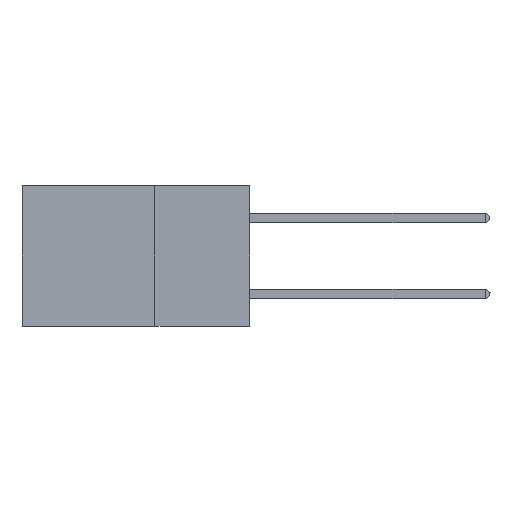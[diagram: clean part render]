
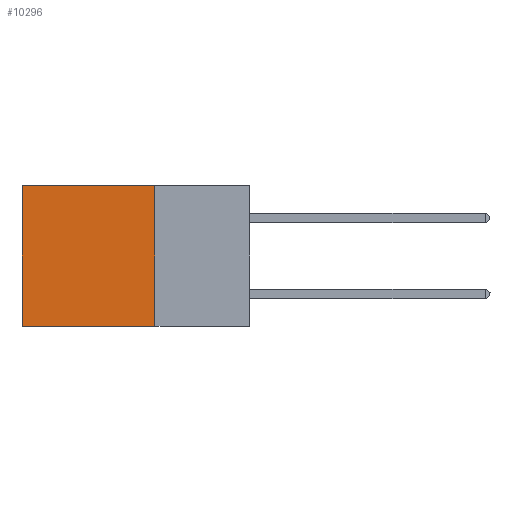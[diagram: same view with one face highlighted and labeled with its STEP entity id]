
A CAD part, left-side view. The second image highlights one B-rep face of the part: STEP entity #10296.
In plain terms, the highlighted planar face has unit normal (-1, 0, 0).
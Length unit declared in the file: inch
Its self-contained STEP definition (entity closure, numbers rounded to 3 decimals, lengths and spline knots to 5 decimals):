
#1873 = LINE ( 'NONE', #22640, #8203 ) ;
#2270 = AXIS2_PLACEMENT_3D ( 'NONE', #21658, #13284, #27161 ) ;
#2515 = CARTESIAN_POINT ( 'NONE',  ( 0.2875, 0.25, -0.37 ) ) ;
#2708 = EDGE_CURVE ( 'NONE', #6858, #5451, #20477, .T. ) ;
#3128 = CARTESIAN_POINT ( 'NONE',  ( 0.2875, 0.25, -0.37 ) ) ;
#3579 = EDGE_CURVE ( 'NONE', #22902, #15163, #1873, .T. ) ;
#5326 = ORIENTED_EDGE ( 'NONE', *, *, #14610, .T. ) ;
#5451 = VERTEX_POINT ( 'NONE', #25141 ) ;
#6858 = VERTEX_POINT ( 'NONE', #11950 ) ;
#7576 = VECTOR ( 'NONE', #18239, 39.37008 ) ;
#8203 = VECTOR ( 'NONE', #26667, 39.37008 ) ;
#9871 = LINE ( 'NONE', #3128, #29063 ) ;
#10122 = EDGE_CURVE ( 'NONE', #15163, #5451, #9871, .T. ) ;
#10296 = ADVANCED_FACE ( 'NONE', ( #26131 ), #12541, .F. ) ;
#11008 = ORIENTED_EDGE ( 'NONE', *, *, #10122, .F. ) ;
#11103 = EDGE_LOOP ( 'NONE', ( #16072, #11008, #27109, #5326 ) ) ;
#11950 = CARTESIAN_POINT ( 'NONE',  ( 0.2875, 0.6, 0. ) ) ;
#12541 = PLANE ( 'NONE',  #2270 ) ;
#13284 = DIRECTION ( 'NONE',  ( 1., 0., 0. ) ) ;
#14610 = EDGE_CURVE ( 'NONE', #22902, #6858, #26478, .T. ) ;
#14829 = DIRECTION ( 'NONE',  ( 0., 1., 0. ) ) ;
#15163 = VERTEX_POINT ( 'NONE', #2515 ) ;
#16072 = ORIENTED_EDGE ( 'NONE', *, *, #2708, .T. ) ;
#18239 = DIRECTION ( 'NONE',  ( 0., 0., -1. ) ) ;
#19338 = CARTESIAN_POINT ( 'NONE',  ( 0.2875, 0.25, 0. ) ) ;
#20477 = LINE ( 'NONE', #22858, #7576 ) ;
#21017 = CARTESIAN_POINT ( 'NONE',  ( 0.2875, 0.25, 0. ) ) ;
#21658 = CARTESIAN_POINT ( 'NONE',  ( 0.2875, 0.25, 0. ) ) ;
#22640 = CARTESIAN_POINT ( 'NONE',  ( 0.2875, 0.25, 0. ) ) ;
#22858 = CARTESIAN_POINT ( 'NONE',  ( 0.2875, 0.6, 0. ) ) ;
#22902 = VERTEX_POINT ( 'NONE', #21017 ) ;
#23474 = VECTOR ( 'NONE', #14829, 39.37008 ) ;
#25141 = CARTESIAN_POINT ( 'NONE',  ( 0.2875, 0.6, -0.37 ) ) ;
#25986 = DIRECTION ( 'NONE',  ( 0., 1., 0. ) ) ;
#26131 = FACE_OUTER_BOUND ( 'NONE', #11103, .T. ) ;
#26478 = LINE ( 'NONE', #19338, #23474 ) ;
#26667 = DIRECTION ( 'NONE',  ( 0., 0., -1. ) ) ;
#27109 = ORIENTED_EDGE ( 'NONE', *, *, #3579, .F. ) ;
#27161 = DIRECTION ( 'NONE',  ( 0., 0., -1. ) ) ;
#29063 = VECTOR ( 'NONE', #25986, 39.37008 ) ;
